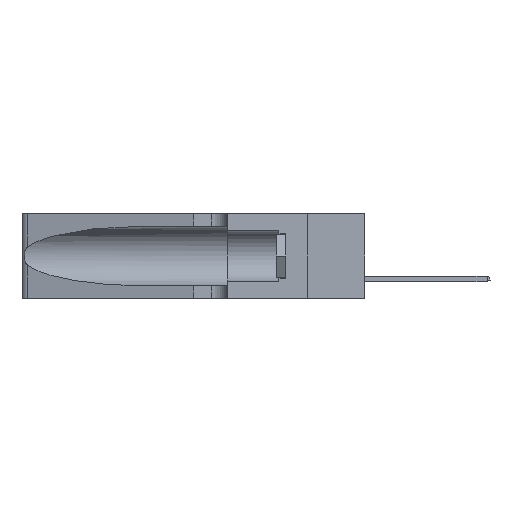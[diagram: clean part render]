
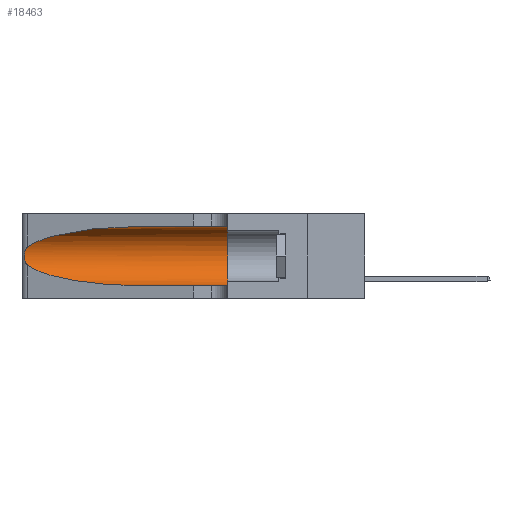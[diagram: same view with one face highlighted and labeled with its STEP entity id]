
A CAD part, left-side view. The second image highlights one B-rep face of the part: STEP entity #18463.
In plain terms, the highlighted cylindrical face has radius 3.308 mm (diameter 6.617 mm), a partial arc.
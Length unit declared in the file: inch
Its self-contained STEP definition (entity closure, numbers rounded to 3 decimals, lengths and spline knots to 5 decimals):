
#492 = DIRECTION ( 'NONE',  ( 0., 0., 1. ) ) ;
#548 = CARTESIAN_POINT ( 'NONE',  ( 0.18966, 0.96281, 0.05475 ) ) ;
#1162 = LINE ( 'NONE', #11686, #29109 ) ;
#1254 =( BOUNDED_CURVE ( )  B_SPLINE_CURVE ( 3, ( #24900, #13513, #13118, #27388 ),
 .UNSPECIFIED., .F., .T. ) 
 B_SPLINE_CURVE_WITH_KNOTS ( ( 4, 4 ),
 ( 1.5708, 2.84003 ),
 .UNSPECIFIED. ) 
 CURVE ( )  GEOMETRIC_REPRESENTATION_ITEM ( )  RATIONAL_B_SPLINE_CURVE ( ( 1., 0.87, 0.87, 1. ) ) 
 REPRESENTATION_ITEM ( '' )  );
#2016 = EDGE_CURVE ( 'NONE', #19762, #27958, #1254, .T. ) ;
#2743 = CARTESIAN_POINT ( 'NONE',  ( 0.1305, 0.35, 0.31525 ) ) ;
#2840 = CARTESIAN_POINT ( 'NONE',  ( 0.1305, 0.35, 0.185 ) ) ;
#3133 = CARTESIAN_POINT ( 'NONE',  ( 0.25487, 1.22718, 0.22369 ) ) ;
#3860 = DIRECTION ( 'NONE',  ( 0., 0., -1. ) ) ;
#4524 = ORIENTED_EDGE ( 'NONE', *, *, #15733, .T. ) ;
#5480 = CARTESIAN_POINT ( 'NONE',  ( 0.26075, 1.23896, 0.19203 ) ) ;
#5794 = EDGE_CURVE ( 'NONE', #27958, #17076, #21480, .T. ) ;
#7041 = CARTESIAN_POINT ( 'NONE',  ( 0.25789, 1.23486, 0.15765 ) ) ;
#7631 = VERTEX_POINT ( 'NONE', #26430 ) ;
#7770 = CARTESIAN_POINT ( 'NONE',  ( 0.25639, 1.23186, 0.15144 ) ) ;
#9339 = ORIENTED_EDGE ( 'NONE', *, *, #5794, .T. ) ;
#9506 = CARTESIAN_POINT ( 'NONE',  ( 0.25487, 1.22718, 0.22369 ) ) ;
#9951 = FACE_OUTER_BOUND ( 'NONE', #22433, .T. ) ;
#9964 = CARTESIAN_POINT ( 'NONE',  ( 0.26018, 1.23835, 0.19895 ) ) ;
#10072 = CARTESIAN_POINT ( 'NONE',  ( 0.25555, 1.22993, 0.14849 ) ) ;
#11199 = VERTEX_POINT ( 'NONE', #18978 ) ;
#11686 = CARTESIAN_POINT ( 'NONE',  ( 0.1305, 1.61858, 0.31525 ) ) ;
#12274 = CARTESIAN_POINT ( 'NONE',  ( 0.1305, 0.72297, 0.05475 ) ) ;
#12574 = EDGE_CURVE ( 'NONE', #17076, #11199, #26534, .T. ) ;
#13118 = CARTESIAN_POINT ( 'NONE',  ( 0.2373, 1.15595, 0.28018 ) ) ;
#13513 = CARTESIAN_POINT ( 'NONE',  ( 0.18966, 0.96281, 0.31525 ) ) ;
#13614 = EDGE_CURVE ( 'NONE', #19762, #19750, #1162, .T. ) ;
#13893 = CARTESIAN_POINT ( 'NONE',  ( 0.25639, 1.23184, 0.21858 ) ) ;
#14368 = CARTESIAN_POINT ( 'NONE',  ( 0.25487, 1.22718, 0.14631 ) ) ;
#14817 = AXIS2_PLACEMENT_3D ( 'NONE', #2840, #21249, #492 ) ;
#14930 = CARTESIAN_POINT ( 'NONE',  ( 0.1305, 1.61858, 0.05475 ) ) ;
#15208 = AXIS2_PLACEMENT_3D ( 'NONE', #24510, #26881, #3860 ) ;
#15733 = EDGE_CURVE ( 'NONE', #11199, #7631, #28324, .T. ) ;
#16281 = CARTESIAN_POINT ( 'NONE',  ( 0.25487, 1.22718, 0.14631 ) ) ;
#17076 = VERTEX_POINT ( 'NONE', #26769 ) ;
#17609 = CYLINDRICAL_SURFACE ( 'NONE', #15208, 0.13025 ) ;
#18463 = ADVANCED_FACE ( 'NONE', ( #9951 ), #17609, .F. ) ;
#18978 = CARTESIAN_POINT ( 'NONE',  ( 0.1305, 0.72297, 0.05475 ) ) ;
#19750 = VERTEX_POINT ( 'NONE', #2743 ) ;
#19762 = VERTEX_POINT ( 'NONE', #26052 ) ;
#20936 = CARTESIAN_POINT ( 'NONE',  ( 0.25555, 1.22994, 0.2215 ) ) ;
#21249 = DIRECTION ( 'NONE',  ( 0., 1., 0. ) ) ;
#21480 = B_SPLINE_CURVE_WITH_KNOTS ( 'NONE', 3,
 ( #3133, #20936, #13893, #23868, #23344, #9964, #5480, #21636, #26244, #28593, #7041, #7770, #10072, #16281 ),
 .UNSPECIFIED., .F., .F.,
 ( 4, 2, 2, 2, 2, 2, 4 ),
 ( 0., 0.00027, 0.00053, 0.00107, 0.0016, 0.00187, 0.00214 ),
 .UNSPECIFIED. ) ;
#21636 = CARTESIAN_POINT ( 'NONE',  ( 0.26075, 1.23896, 0.178 ) ) ;
#22433 = EDGE_LOOP ( 'NONE', ( #28612, #9339, #27443, #4524, #23146, #27876 ) ) ;
#22730 = EDGE_CURVE ( 'NONE', #19750, #7631, #29166, .T. ) ;
#23146 = ORIENTED_EDGE ( 'NONE', *, *, #22730, .F. ) ;
#23344 = CARTESIAN_POINT ( 'NONE',  ( 0.25854, 1.2359, 0.20912 ) ) ;
#23868 = CARTESIAN_POINT ( 'NONE',  ( 0.25787, 1.23484, 0.2124 ) ) ;
#24267 = VECTOR ( 'NONE', #26362, 39.37008 ) ;
#24510 = CARTESIAN_POINT ( 'NONE',  ( 0.1305, 1.61858, 0.185 ) ) ;
#24900 = CARTESIAN_POINT ( 'NONE',  ( 0.1305, 0.72297, 0.31525 ) ) ;
#26052 = CARTESIAN_POINT ( 'NONE',  ( 0.1305, 0.72297, 0.31525 ) ) ;
#26202 = CARTESIAN_POINT ( 'NONE',  ( 0.2373, 1.15595, 0.08982 ) ) ;
#26244 = CARTESIAN_POINT ( 'NONE',  ( 0.26017, 1.23833, 0.17102 ) ) ;
#26362 = DIRECTION ( 'NONE',  ( 0., -1., 0. ) ) ;
#26430 = CARTESIAN_POINT ( 'NONE',  ( 0.1305, 0.35, 0.05475 ) ) ;
#26534 =( BOUNDED_CURVE ( )  B_SPLINE_CURVE ( 3, ( #14368, #26202, #548, #12274 ),
 .UNSPECIFIED., .F., .F. ) 
 B_SPLINE_CURVE_WITH_KNOTS ( ( 4, 4 ),
 ( 3.44316, 4.71239 ),
 .UNSPECIFIED. ) 
 CURVE ( )  GEOMETRIC_REPRESENTATION_ITEM ( )  RATIONAL_B_SPLINE_CURVE ( ( 1., 0.87, 0.87, 1. ) ) 
 REPRESENTATION_ITEM ( '' )  );
#26769 = CARTESIAN_POINT ( 'NONE',  ( 0.25487, 1.22718, 0.14631 ) ) ;
#26881 = DIRECTION ( 'NONE',  ( 0., -1., 0. ) ) ;
#27388 = CARTESIAN_POINT ( 'NONE',  ( 0.25487, 1.22718, 0.22369 ) ) ;
#27443 = ORIENTED_EDGE ( 'NONE', *, *, #12574, .T. ) ;
#27876 = ORIENTED_EDGE ( 'NONE', *, *, #13614, .F. ) ;
#27958 = VERTEX_POINT ( 'NONE', #9506 ) ;
#28324 = LINE ( 'NONE', #14930, #24267 ) ;
#28593 = CARTESIAN_POINT ( 'NONE',  ( 0.25856, 1.23593, 0.16098 ) ) ;
#28612 = ORIENTED_EDGE ( 'NONE', *, *, #2016, .T. ) ;
#29109 = VECTOR ( 'NONE', #29761, 39.37008 ) ;
#29166 = CIRCLE ( 'NONE', #14817, 0.13025 ) ;
#29761 = DIRECTION ( 'NONE',  ( 0., -1., 0. ) ) ;
